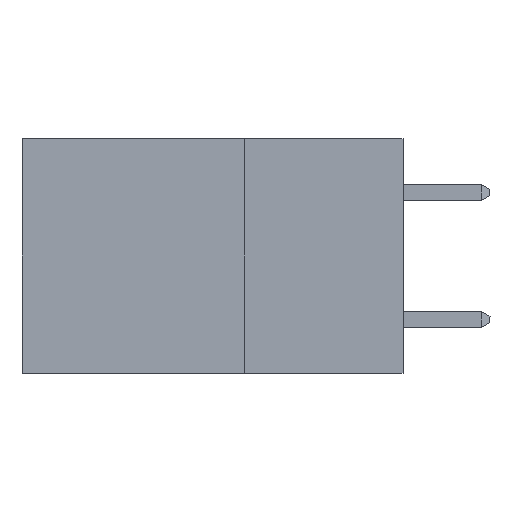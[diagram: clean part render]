
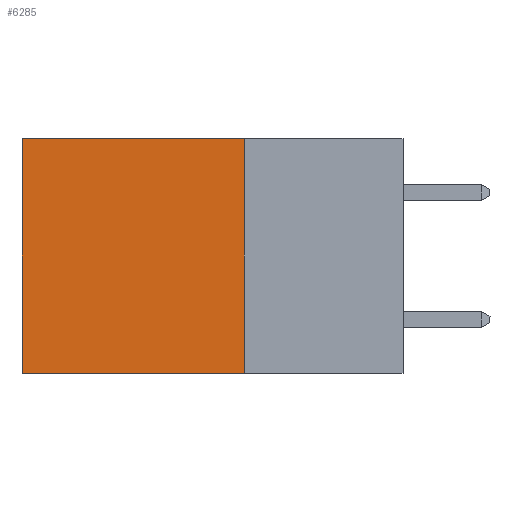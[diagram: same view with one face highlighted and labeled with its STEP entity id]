
A CAD part, left-side view. The second image highlights one B-rep face of the part: STEP entity #6285.
In plain terms, the highlighted planar face has unit normal (-1, 0, 0).
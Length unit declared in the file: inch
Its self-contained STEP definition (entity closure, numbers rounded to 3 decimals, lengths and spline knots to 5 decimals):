
#70 = DIRECTION ( 'NONE',  ( 0., 0., -1. ) ) ;
#673 = VECTOR ( 'NONE', #11037, 39.37008 ) ;
#957 = AXIS2_PLACEMENT_3D ( 'NONE', #1976, #9610, #70 ) ;
#1217 = VERTEX_POINT ( 'NONE', #5565 ) ;
#1375 = LINE ( 'NONE', #4694, #673 ) ;
#1787 = CARTESIAN_POINT ( 'NONE',  ( 0.2875, 0.25, -0.37 ) ) ;
#1879 = EDGE_CURVE ( 'NONE', #1217, #7322, #2740, .T. ) ;
#1976 = CARTESIAN_POINT ( 'NONE',  ( 0.2875, 0.25, 0. ) ) ;
#2217 = DIRECTION ( 'NONE',  ( 0., 0., -1. ) ) ;
#2740 = LINE ( 'NONE', #2798, #6409 ) ;
#2798 = CARTESIAN_POINT ( 'NONE',  ( 0.2875, 0.25, 0. ) ) ;
#2825 = FACE_OUTER_BOUND ( 'NONE', #4767, .T. ) ;
#4364 = ORIENTED_EDGE ( 'NONE', *, *, #7185, .F. ) ;
#4694 = CARTESIAN_POINT ( 'NONE',  ( 0.2875, 0.6, 0. ) ) ;
#4767 = EDGE_LOOP ( 'NONE', ( #10641, #4364, #5887, #7762 ) ) ;
#5110 = VERTEX_POINT ( 'NONE', #11214 ) ;
#5565 = CARTESIAN_POINT ( 'NONE',  ( 0.2875, 0.25, 0. ) ) ;
#5887 = ORIENTED_EDGE ( 'NONE', *, *, #6733, .F. ) ;
#6285 = ADVANCED_FACE ( 'NONE', ( #2825 ), #6325, .F. ) ;
#6325 = PLANE ( 'NONE',  #957 ) ;
#6409 = VECTOR ( 'NONE', #8857, 39.37008 ) ;
#6733 = EDGE_CURVE ( 'NONE', #1217, #10919, #10055, .T. ) ;
#7185 = EDGE_CURVE ( 'NONE', #10919, #5110, #7630, .T. ) ;
#7322 = VERTEX_POINT ( 'NONE', #9641 ) ;
#7536 = CARTESIAN_POINT ( 'NONE',  ( 0.2875, 0.25, 0. ) ) ;
#7630 = LINE ( 'NONE', #9408, #8079 ) ;
#7682 = DIRECTION ( 'NONE',  ( 0., 1., 0. ) ) ;
#7762 = ORIENTED_EDGE ( 'NONE', *, *, #1879, .T. ) ;
#8079 = VECTOR ( 'NONE', #7682, 39.37008 ) ;
#8857 = DIRECTION ( 'NONE',  ( 0., 1., 0. ) ) ;
#9172 = VECTOR ( 'NONE', #2217, 39.37008 ) ;
#9408 = CARTESIAN_POINT ( 'NONE',  ( 0.2875, 0.25, -0.37 ) ) ;
#9610 = DIRECTION ( 'NONE',  ( 1., 0., 0. ) ) ;
#9641 = CARTESIAN_POINT ( 'NONE',  ( 0.2875, 0.6, 0. ) ) ;
#10055 = LINE ( 'NONE', #7536, #9172 ) ;
#10641 = ORIENTED_EDGE ( 'NONE', *, *, #11266, .T. ) ;
#10919 = VERTEX_POINT ( 'NONE', #1787 ) ;
#11037 = DIRECTION ( 'NONE',  ( 0., 0., -1. ) ) ;
#11214 = CARTESIAN_POINT ( 'NONE',  ( 0.2875, 0.6, -0.37 ) ) ;
#11266 = EDGE_CURVE ( 'NONE', #7322, #5110, #1375, .T. ) ;
